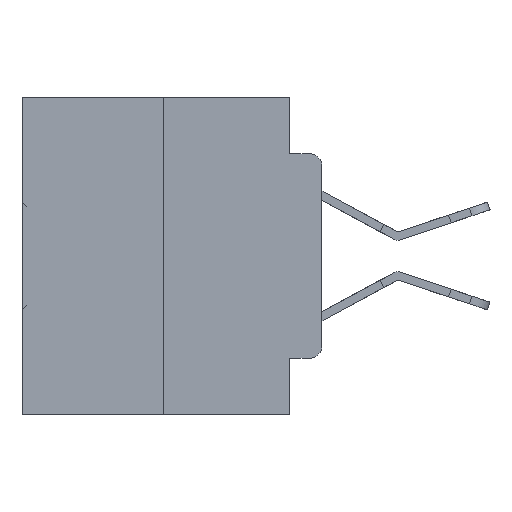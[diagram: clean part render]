
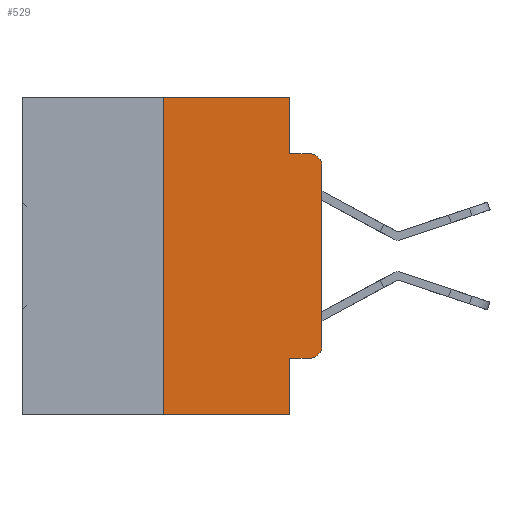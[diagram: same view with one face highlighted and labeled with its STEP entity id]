
A CAD part, left-side view. The second image highlights one B-rep face of the part: STEP entity #529.
In plain terms, the highlighted planar face has unit normal (-1, 0, 0).
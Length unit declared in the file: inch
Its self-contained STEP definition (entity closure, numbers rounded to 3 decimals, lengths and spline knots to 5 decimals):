
#454 = LINE ( 'NONE', #6468, #14250 ) ;
#529 = ADVANCED_FACE ( 'NONE', ( #22238 ), #3877, .F. ) ;
#627 = VECTOR ( 'NONE', #30460, 39.37008 ) ;
#1015 = CARTESIAN_POINT ( 'NONE',  ( 0., 0.25, 0. ) ) ;
#1022 = EDGE_CURVE ( 'NONE', #17005, #16612, #15134, .T. ) ;
#2138 = LINE ( 'NONE', #28083, #8657 ) ;
#2848 = CARTESIAN_POINT ( 'NONE',  ( 0., 0.051, -0.4115 ) ) ;
#3877 = PLANE ( 'NONE',  #8612 ) ;
#4757 = VERTEX_POINT ( 'NONE', #5405 ) ;
#4779 = ORIENTED_EDGE ( 'NONE', *, *, #9369, .T. ) ;
#5018 = EDGE_CURVE ( 'NONE', #21103, #4757, #28305, .T. ) ;
#5288 = EDGE_CURVE ( 'NONE', #21094, #29822, #15423, .T. ) ;
#5405 = CARTESIAN_POINT ( 'NONE',  ( 0., 0., -0.1085 ) ) ;
#5456 = EDGE_CURVE ( 'NONE', #29822, #19141, #9441, .T. ) ;
#6468 = CARTESIAN_POINT ( 'NONE',  ( 0., 0.473, 0. ) ) ;
#6608 = VECTOR ( 'NONE', #9390, 39.37008 ) ;
#7389 = ORIENTED_EDGE ( 'NONE', *, *, #15337, .T. ) ;
#7668 = ORIENTED_EDGE ( 'NONE', *, *, #11909, .F. ) ;
#7891 = VECTOR ( 'NONE', #28738, 39.37008 ) ;
#8023 = LINE ( 'NONE', #27827, #627 ) ;
#8612 = AXIS2_PLACEMENT_3D ( 'NONE', #25597, #34351, #9614 ) ;
#8657 = VECTOR ( 'NONE', #12032, 39.37008 ) ;
#9369 = EDGE_CURVE ( 'NONE', #4757, #19141, #14880, .T. ) ;
#9390 = DIRECTION ( 'NONE',  ( 0., 0., 1. ) ) ;
#9441 = LINE ( 'NONE', #28613, #15831 ) ;
#9614 = DIRECTION ( 'NONE',  ( 0., 0., -1. ) ) ;
#10414 = VERTEX_POINT ( 'NONE', #15878 ) ;
#10972 = DIRECTION ( 'NONE',  ( 0., 0., 1. ) ) ;
#11130 = AXIS2_PLACEMENT_3D ( 'NONE', #29020, #13119, #31655 ) ;
#11592 = CARTESIAN_POINT ( 'NONE',  ( 0., 0.25, 0. ) ) ;
#11909 = EDGE_CURVE ( 'NONE', #10414, #14564, #13903, .T. ) ;
#12032 = DIRECTION ( 'NONE',  ( 0., -1., 0. ) ) ;
#13119 = DIRECTION ( 'NONE',  ( -1., 0., 0. ) ) ;
#13903 = LINE ( 'NONE', #1015, #6608 ) ;
#14250 = VECTOR ( 'NONE', #17419, 39.37008 ) ;
#14424 = DIRECTION ( 'NONE',  ( -1., 0., 0. ) ) ;
#14564 = VERTEX_POINT ( 'NONE', #11592 ) ;
#14642 = CARTESIAN_POINT ( 'NONE',  ( 0., 0., 0. ) ) ;
#14880 = CIRCLE ( 'NONE', #24576, 0.02 ) ;
#15064 = CARTESIAN_POINT ( 'NONE',  ( 0., 0.051, 0. ) ) ;
#15134 = LINE ( 'NONE', #15064, #7891 ) ;
#15260 = ORIENTED_EDGE ( 'NONE', *, *, #5288, .F. ) ;
#15337 = EDGE_CURVE ( 'NONE', #10414, #16612, #2138, .T. ) ;
#15423 = LINE ( 'NONE', #20054, #27867 ) ;
#15828 = EDGE_LOOP ( 'NONE', ( #21832, #4779, #33550, #15260, #17454, #7668, #7389, #33281, #26308, #17580 ) ) ;
#15831 = VECTOR ( 'NONE', #31242, 39.37008 ) ;
#15878 = CARTESIAN_POINT ( 'NONE',  ( 0., 0.25, -0.5 ) ) ;
#16612 = VERTEX_POINT ( 'NONE', #23043 ) ;
#17005 = VERTEX_POINT ( 'NONE', #2848 ) ;
#17419 = DIRECTION ( 'NONE',  ( 0., -1., 0. ) ) ;
#17454 = ORIENTED_EDGE ( 'NONE', *, *, #22475, .F. ) ;
#17515 = DIRECTION ( 'NONE',  ( 0., 0., -1. ) ) ;
#17580 = ORIENTED_EDGE ( 'NONE', *, *, #27323, .T. ) ;
#19141 = VERTEX_POINT ( 'NONE', #30564 ) ;
#19803 = CARTESIAN_POINT ( 'NONE',  ( 0., 0., -0.3915 ) ) ;
#20054 = CARTESIAN_POINT ( 'NONE',  ( 0., 0.051, 0. ) ) ;
#21094 = VERTEX_POINT ( 'NONE', #22499 ) ;
#21103 = VERTEX_POINT ( 'NONE', #19803 ) ;
#21832 = ORIENTED_EDGE ( 'NONE', *, *, #5018, .T. ) ;
#22238 = FACE_OUTER_BOUND ( 'NONE', #15828, .T. ) ;
#22475 = EDGE_CURVE ( 'NONE', #14564, #21094, #454, .T. ) ;
#22499 = CARTESIAN_POINT ( 'NONE',  ( 0., 0.051, 0. ) ) ;
#23043 = CARTESIAN_POINT ( 'NONE',  ( 0., 0.051, -0.5 ) ) ;
#23093 = CARTESIAN_POINT ( 'NONE',  ( 0., 0.051, -0.0885 ) ) ;
#24576 = AXIS2_PLACEMENT_3D ( 'NONE', #30298, #14424, #32939 ) ;
#25597 = CARTESIAN_POINT ( 'NONE',  ( 0., 0.473, 0. ) ) ;
#25776 = EDGE_CURVE ( 'NONE', #17005, #27924, #8023, .T. ) ;
#26308 = ORIENTED_EDGE ( 'NONE', *, *, #25776, .T. ) ;
#26699 = CARTESIAN_POINT ( 'NONE',  ( 0., 0.02, -0.4115 ) ) ;
#26828 = CIRCLE ( 'NONE', #11130, 0.02 ) ;
#27323 = EDGE_CURVE ( 'NONE', #27924, #21103, #26828, .T. ) ;
#27827 = CARTESIAN_POINT ( 'NONE',  ( 0., 0.051, -0.4115 ) ) ;
#27867 = VECTOR ( 'NONE', #17515, 39.37008 ) ;
#27924 = VERTEX_POINT ( 'NONE', #26699 ) ;
#28083 = CARTESIAN_POINT ( 'NONE',  ( 0., 0.473, -0.5 ) ) ;
#28305 = LINE ( 'NONE', #14642, #34465 ) ;
#28613 = CARTESIAN_POINT ( 'NONE',  ( 0., 0.051, -0.0885 ) ) ;
#28738 = DIRECTION ( 'NONE',  ( 0., 0., -1. ) ) ;
#29020 = CARTESIAN_POINT ( 'NONE',  ( 0., 0.02, -0.3915 ) ) ;
#29822 = VERTEX_POINT ( 'NONE', #23093 ) ;
#30298 = CARTESIAN_POINT ( 'NONE',  ( 0., 0.02, -0.1085 ) ) ;
#30460 = DIRECTION ( 'NONE',  ( 0., -1., 0. ) ) ;
#30564 = CARTESIAN_POINT ( 'NONE',  ( 0., 0.02, -0.0885 ) ) ;
#31242 = DIRECTION ( 'NONE',  ( 0., -1., 0. ) ) ;
#31655 = DIRECTION ( 'NONE',  ( 0., 0., -1. ) ) ;
#32939 = DIRECTION ( 'NONE',  ( 0., 0., -1. ) ) ;
#33281 = ORIENTED_EDGE ( 'NONE', *, *, #1022, .F. ) ;
#33550 = ORIENTED_EDGE ( 'NONE', *, *, #5456, .F. ) ;
#34351 = DIRECTION ( 'NONE',  ( 1., 0., 0. ) ) ;
#34465 = VECTOR ( 'NONE', #10972, 39.37008 ) ;
